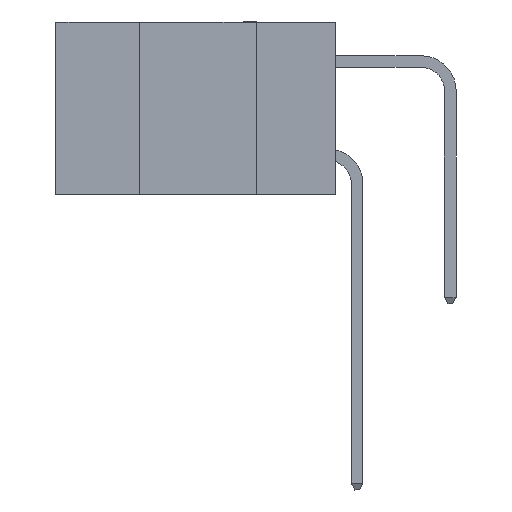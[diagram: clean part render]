
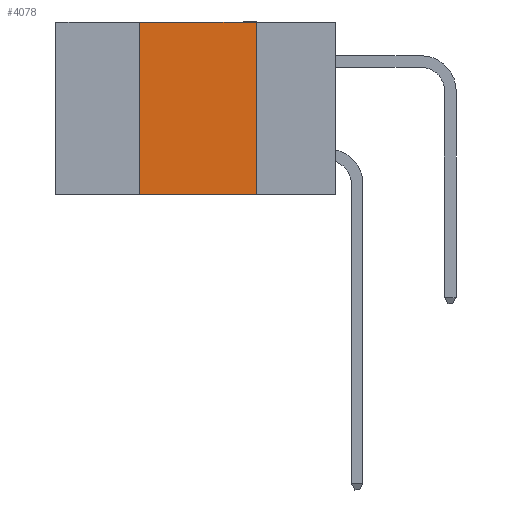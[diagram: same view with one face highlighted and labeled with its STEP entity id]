
A CAD part, left-side view. The second image highlights one B-rep face of the part: STEP entity #4078.
In plain terms, the highlighted planar face has unit normal (-1, 0, 0).
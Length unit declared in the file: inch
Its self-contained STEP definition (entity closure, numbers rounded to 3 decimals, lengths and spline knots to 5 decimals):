
#159 = VECTOR ( 'NONE', #5322, 39.37008 ) ;
#444 = EDGE_CURVE ( 'NONE', #18880, #17851, #5441, .T. ) ;
#910 = LINE ( 'NONE', #13467, #159 ) ;
#956 = CARTESIAN_POINT ( 'NONE',  ( 0., 0.42, 0. ) ) ;
#2485 = FACE_OUTER_BOUND ( 'NONE', #8929, .T. ) ;
#2654 = VECTOR ( 'NONE', #6131, 39.37008 ) ;
#3443 = ORIENTED_EDGE ( 'NONE', *, *, #444, .F. ) ;
#3598 = CARTESIAN_POINT ( 'NONE',  ( 0., 0.17, 0. ) ) ;
#3805 = DIRECTION ( 'NONE',  ( 0., -1., 0. ) ) ;
#4078 = ADVANCED_FACE ( 'NONE', ( #2485 ), #19655, .F. ) ;
#4695 = CARTESIAN_POINT ( 'NONE',  ( 0., 0.17, -0.37 ) ) ;
#4851 = DIRECTION ( 'NONE',  ( 0., 0., -1. ) ) ;
#5322 = DIRECTION ( 'NONE',  ( 0., -1., 0. ) ) ;
#5441 = LINE ( 'NONE', #956, #2654 ) ;
#6131 = DIRECTION ( 'NONE',  ( 0., 0., 1. ) ) ;
#7046 = AXIS2_PLACEMENT_3D ( 'NONE', #8219, #14856, #4851 ) ;
#7614 = ORIENTED_EDGE ( 'NONE', *, *, #14671, .F. ) ;
#7856 = ORIENTED_EDGE ( 'NONE', *, *, #9197, .F. ) ;
#8219 = CARTESIAN_POINT ( 'NONE',  ( 0., 0.6, 0. ) ) ;
#8311 = VERTEX_POINT ( 'NONE', #3598 ) ;
#8395 = VECTOR ( 'NONE', #18128, 39.37008 ) ;
#8929 = EDGE_LOOP ( 'NONE', ( #7614, #7856, #3443, #9619 ) ) ;
#9197 = EDGE_CURVE ( 'NONE', #17851, #8311, #12279, .T. ) ;
#9619 = ORIENTED_EDGE ( 'NONE', *, *, #16926, .T. ) ;
#11610 = CARTESIAN_POINT ( 'NONE',  ( 0., 0.6, 0. ) ) ;
#12038 = VECTOR ( 'NONE', #3805, 39.37008 ) ;
#12279 = LINE ( 'NONE', #11610, #12038 ) ;
#13467 = CARTESIAN_POINT ( 'NONE',  ( 0., 0.6, -0.37 ) ) ;
#14451 = CARTESIAN_POINT ( 'NONE',  ( 0., 0.42, 0. ) ) ;
#14518 = VERTEX_POINT ( 'NONE', #4695 ) ;
#14671 = EDGE_CURVE ( 'NONE', #8311, #14518, #16311, .T. ) ;
#14856 = DIRECTION ( 'NONE',  ( 1., 0., 0. ) ) ;
#16311 = LINE ( 'NONE', #18052, #8395 ) ;
#16926 = EDGE_CURVE ( 'NONE', #18880, #14518, #910, .T. ) ;
#17325 = CARTESIAN_POINT ( 'NONE',  ( 0., 0.42, -0.37 ) ) ;
#17851 = VERTEX_POINT ( 'NONE', #14451 ) ;
#18052 = CARTESIAN_POINT ( 'NONE',  ( 0., 0.17, 0. ) ) ;
#18128 = DIRECTION ( 'NONE',  ( 0., 0., -1. ) ) ;
#18880 = VERTEX_POINT ( 'NONE', #17325 ) ;
#19655 = PLANE ( 'NONE',  #7046 ) ;
